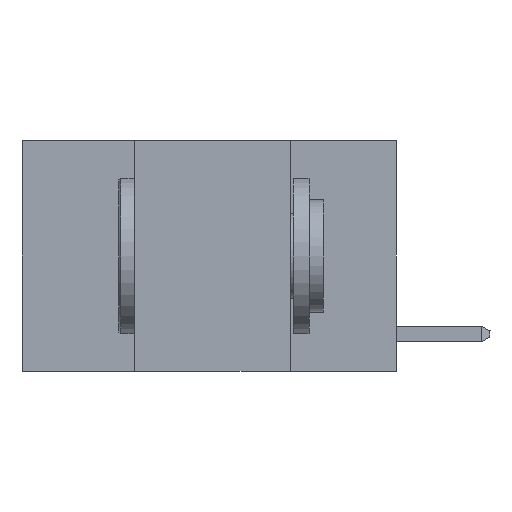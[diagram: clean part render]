
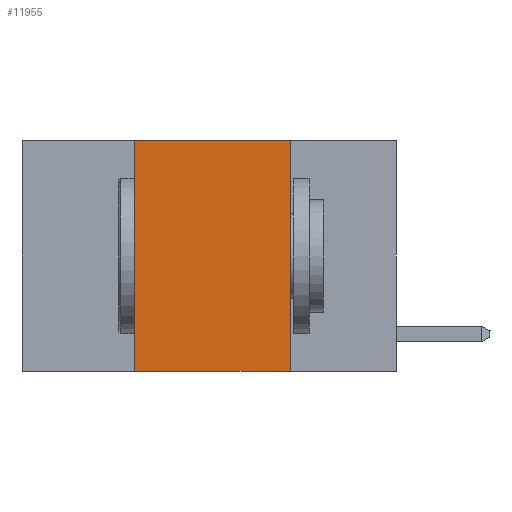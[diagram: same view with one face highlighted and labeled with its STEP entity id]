
A CAD part, left-side view. The second image highlights one B-rep face of the part: STEP entity #11955.
In plain terms, the highlighted planar face has unit normal (-1, 0, 0).
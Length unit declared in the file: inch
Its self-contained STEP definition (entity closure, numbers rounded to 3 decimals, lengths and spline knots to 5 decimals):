
#211 = DIRECTION ( 'NONE',  ( 0., 0., -1. ) ) ;
#366 = LINE ( 'NONE', #28498, #2804 ) ;
#974 = DIRECTION ( 'NONE',  ( 0., 0., -1. ) ) ;
#990 = DIRECTION ( 'NONE',  ( 0., -1., 0. ) ) ;
#1141 = CARTESIAN_POINT ( 'NONE',  ( 0., 0.6, 0. ) ) ;
#2804 = VECTOR ( 'NONE', #211, 39.37008 ) ;
#6046 = VECTOR ( 'NONE', #21833, 39.37008 ) ;
#6822 = VECTOR ( 'NONE', #6881, 39.37008 ) ;
#6881 = DIRECTION ( 'NONE',  ( 0., 0., 1. ) ) ;
#9081 = ORIENTED_EDGE ( 'NONE', *, *, #11794, .F. ) ;
#11441 = ORIENTED_EDGE ( 'NONE', *, *, #26873, .T. ) ;
#11794 = EDGE_CURVE ( 'NONE', #18931, #29809, #25856, .T. ) ;
#11955 = ADVANCED_FACE ( 'NONE', ( #19766 ), #29248, .F. ) ;
#12151 = CARTESIAN_POINT ( 'NONE',  ( 0., 0.42, 0. ) ) ;
#13071 = VERTEX_POINT ( 'NONE', #14639 ) ;
#13267 = AXIS2_PLACEMENT_3D ( 'NONE', #17444, #15092, #974 ) ;
#14639 = CARTESIAN_POINT ( 'NONE',  ( 0., 0.17, 0. ) ) ;
#14965 = LINE ( 'NONE', #1141, #6046 ) ;
#15092 = DIRECTION ( 'NONE',  ( 1., 0., 0. ) ) ;
#17444 = CARTESIAN_POINT ( 'NONE',  ( 0., 0.6, 0. ) ) ;
#18156 = EDGE_CURVE ( 'NONE', #29809, #13071, #14965, .T. ) ;
#18931 = VERTEX_POINT ( 'NONE', #19417 ) ;
#19417 = CARTESIAN_POINT ( 'NONE',  ( 0., 0.42, -0.37 ) ) ;
#19766 = FACE_OUTER_BOUND ( 'NONE', #30052, .T. ) ;
#20081 = LINE ( 'NONE', #24312, #30604 ) ;
#20164 = VERTEX_POINT ( 'NONE', #25817 ) ;
#21833 = DIRECTION ( 'NONE',  ( 0., -1., 0. ) ) ;
#24312 = CARTESIAN_POINT ( 'NONE',  ( 0., 0.6, -0.37 ) ) ;
#25817 = CARTESIAN_POINT ( 'NONE',  ( 0., 0.17, -0.37 ) ) ;
#25856 = LINE ( 'NONE', #12151, #6822 ) ;
#26751 = EDGE_CURVE ( 'NONE', #13071, #20164, #366, .T. ) ;
#26873 = EDGE_CURVE ( 'NONE', #18931, #20164, #20081, .T. ) ;
#27656 = ORIENTED_EDGE ( 'NONE', *, *, #18156, .F. ) ;
#28498 = CARTESIAN_POINT ( 'NONE',  ( 0., 0.17, 0. ) ) ;
#29248 = PLANE ( 'NONE',  #13267 ) ;
#29809 = VERTEX_POINT ( 'NONE', #30386 ) ;
#30052 = EDGE_LOOP ( 'NONE', ( #30068, #27656, #9081, #11441 ) ) ;
#30068 = ORIENTED_EDGE ( 'NONE', *, *, #26751, .F. ) ;
#30386 = CARTESIAN_POINT ( 'NONE',  ( 0., 0.42, 0. ) ) ;
#30604 = VECTOR ( 'NONE', #990, 39.37008 ) ;
